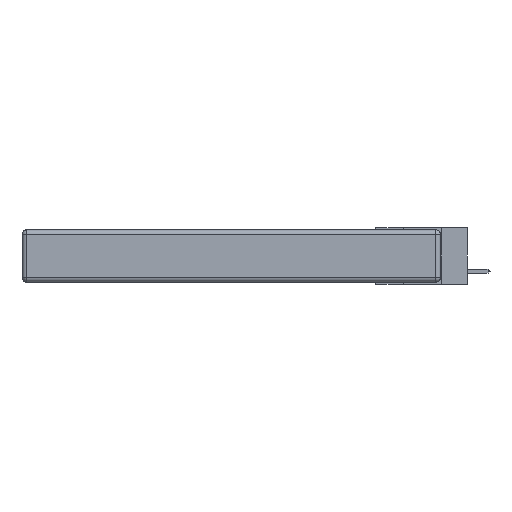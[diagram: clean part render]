
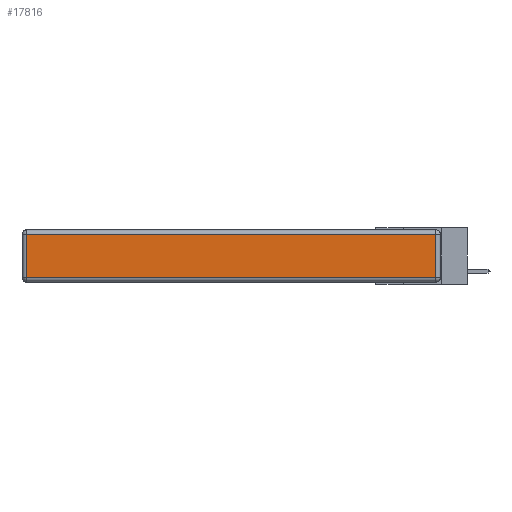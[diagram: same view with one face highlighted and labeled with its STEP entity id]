
A CAD part, left-side view. The second image highlights one B-rep face of the part: STEP entity #17816.
In plain terms, the highlighted planar face has unit normal (-1, 0, 0).
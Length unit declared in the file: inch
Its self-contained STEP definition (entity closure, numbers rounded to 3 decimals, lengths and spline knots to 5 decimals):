
#17 = DIRECTION ( 'NONE',  ( 0., 0., 1. ) ) ;
#3342 = EDGE_CURVE ( 'NONE', #32199, #30541, #28871, .T. ) ;
#4282 = VECTOR ( 'NONE', #18112, 39.37008 ) ;
#5057 = PLANE ( 'NONE',  #6368 ) ;
#5600 = VECTOR ( 'NONE', #8658, 39.37008 ) ;
#5604 = DIRECTION ( 'NONE',  ( 0., 1., 0. ) ) ;
#6368 = AXIS2_PLACEMENT_3D ( 'NONE', #30434, #15269, #17 ) ;
#7297 = DIRECTION ( 'NONE',  ( 0., 0., -1. ) ) ;
#8044 = EDGE_LOOP ( 'NONE', ( #22837, #27638, #10404, #24883 ) ) ;
#8658 = DIRECTION ( 'NONE',  ( 0., 0., 1. ) ) ;
#10271 = VECTOR ( 'NONE', #7297, 39.37008 ) ;
#10404 = ORIENTED_EDGE ( 'NONE', *, *, #31900, .T. ) ;
#10454 = CARTESIAN_POINT ( 'NONE',  ( 0., 0., -0.313 ) ) ;
#13833 = CARTESIAN_POINT ( 'NONE',  ( 0., 2.72, -0.313 ) ) ;
#15031 = LINE ( 'NONE', #22469, #10271 ) ;
#15269 = DIRECTION ( 'NONE',  ( -1., 0., 0. ) ) ;
#15669 = VECTOR ( 'NONE', #5604, 39.37008 ) ;
#17816 = ADVANCED_FACE ( 'NONE', ( #18592 ), #5057, .T. ) ;
#18112 = DIRECTION ( 'NONE',  ( 0., -1., 0. ) ) ;
#18188 = CARTESIAN_POINT ( 'NONE',  ( 0., 0.03, -0.03 ) ) ;
#18592 = FACE_OUTER_BOUND ( 'NONE', #8044, .T. ) ;
#20816 = CARTESIAN_POINT ( 'NONE',  ( 0., 2.75, -0.03 ) ) ;
#21300 = VERTEX_POINT ( 'NONE', #18188 ) ;
#22469 = CARTESIAN_POINT ( 'NONE',  ( 0., 2.72, -0.343 ) ) ;
#22837 = ORIENTED_EDGE ( 'NONE', *, *, #3342, .T. ) ;
#23044 = CARTESIAN_POINT ( 'NONE',  ( 0., 0.03, -0.313 ) ) ;
#24004 = LINE ( 'NONE', #20816, #15669 ) ;
#24883 = ORIENTED_EDGE ( 'NONE', *, *, #26404, .T. ) ;
#26158 = CARTESIAN_POINT ( 'NONE',  ( 0., 0.03, -0.343 ) ) ;
#26404 = EDGE_CURVE ( 'NONE', #31459, #32199, #15031, .T. ) ;
#27638 = ORIENTED_EDGE ( 'NONE', *, *, #30037, .T. ) ;
#28871 = LINE ( 'NONE', #10454, #4282 ) ;
#30037 = EDGE_CURVE ( 'NONE', #30541, #21300, #32625, .T. ) ;
#30434 = CARTESIAN_POINT ( 'NONE',  ( 0., 0., -0.343 ) ) ;
#30541 = VERTEX_POINT ( 'NONE', #23044 ) ;
#31459 = VERTEX_POINT ( 'NONE', #32398 ) ;
#31900 = EDGE_CURVE ( 'NONE', #21300, #31459, #24004, .T. ) ;
#32199 = VERTEX_POINT ( 'NONE', #13833 ) ;
#32398 = CARTESIAN_POINT ( 'NONE',  ( 0., 2.72, -0.03 ) ) ;
#32625 = LINE ( 'NONE', #26158, #5600 ) ;
